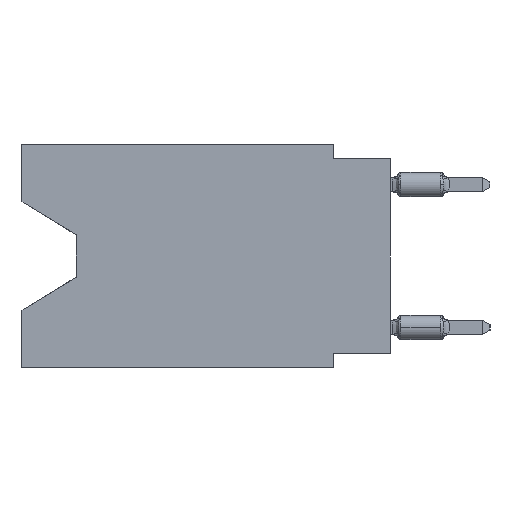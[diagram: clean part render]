
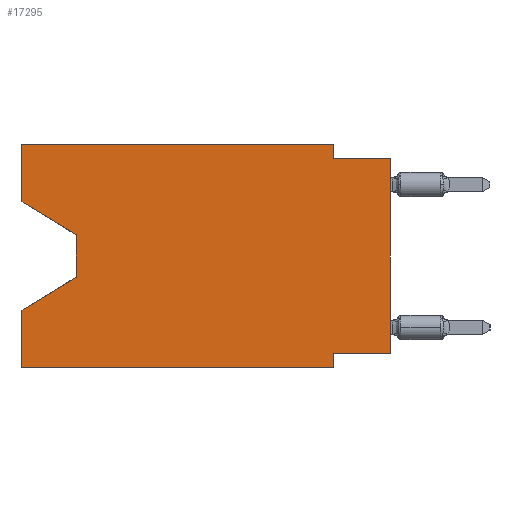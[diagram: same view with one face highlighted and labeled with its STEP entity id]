
A CAD part, left-side view. The second image highlights one B-rep face of the part: STEP entity #17295.
In plain terms, the highlighted planar face has unit normal (-1, 0, 0).
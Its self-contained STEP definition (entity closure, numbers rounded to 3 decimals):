
#108 = LINE ( 'NONE', #28120, #37864 ) ;
#518 = DIRECTION ( 'NONE',  ( 0., 0.855, -0.519 ) ) ;
#719 = DIRECTION ( 'NONE',  ( 1., 0., 0. ) ) ;
#915 = EDGE_CURVE ( 'NONE', #39426, #42097, #6991, .T. ) ;
#1503 = ORIENTED_EDGE ( 'NONE', *, *, #33979, .T. ) ;
#1703 = VECTOR ( 'NONE', #30741, 1000. ) ;
#4062 = ORIENTED_EDGE ( 'NONE', *, *, #31071, .F. ) ;
#4151 = VERTEX_POINT ( 'NONE', #44244 ) ;
#4306 = CARTESIAN_POINT ( 'NONE',  ( 0., 16.383, 0. ) ) ;
#4831 = CARTESIAN_POINT ( 'NONE',  ( 0., 16.383, 0. ) ) ;
#5642 = EDGE_CURVE ( 'NONE', #6560, #11931, #108, .T. ) ;
#6140 = LINE ( 'NONE', #20152, #36216 ) ;
#6560 = VERTEX_POINT ( 'NONE', #17883 ) ;
#6873 = ORIENTED_EDGE ( 'NONE', *, *, #22415, .T. ) ;
#6991 = LINE ( 'NONE', #17326, #15964 ) ;
#7248 = DIRECTION ( 'NONE',  ( 0., 0., 1. ) ) ;
#7378 = DIRECTION ( 'NONE',  ( 0., 0., -1. ) ) ;
#7526 = VECTOR ( 'NONE', #518, 1000. ) ;
#8379 = DIRECTION ( 'NONE',  ( 0., 0., 1. ) ) ;
#8474 = CARTESIAN_POINT ( 'NONE',  ( 0., 16.383, -9.906 ) ) ;
#8955 = DIRECTION ( 'NONE',  ( 0., -1., 0. ) ) ;
#9153 = ORIENTED_EDGE ( 'NONE', *, *, #14488, .F. ) ;
#10204 = CARTESIAN_POINT ( 'NONE',  ( 0., 2.54, -0.635 ) ) ;
#10482 = VECTOR ( 'NONE', #43753, 1000. ) ;
#10661 = VECTOR ( 'NONE', #20862, 1000. ) ;
#11818 = LINE ( 'NONE', #39403, #36347 ) ;
#11931 = VERTEX_POINT ( 'NONE', #4306 ) ;
#12626 = LINE ( 'NONE', #4831, #39075 ) ;
#13774 = ORIENTED_EDGE ( 'NONE', *, *, #33832, .F. ) ;
#13860 = EDGE_CURVE ( 'NONE', #42097, #24738, #31935, .T. ) ;
#14488 = EDGE_CURVE ( 'NONE', #4151, #15485, #6140, .T. ) ;
#15102 = CARTESIAN_POINT ( 'NONE',  ( 0., 2.54, -9.906 ) ) ;
#15473 = LINE ( 'NONE', #37067, #10482 ) ;
#15485 = VERTEX_POINT ( 'NONE', #10204 ) ;
#15964 = VECTOR ( 'NONE', #38912, 1000. ) ;
#16882 = AXIS2_PLACEMENT_3D ( 'NONE', #36060, #719, #7378 ) ;
#17088 = DIRECTION ( 'NONE',  ( 0., 0., -1. ) ) ;
#17162 = ORIENTED_EDGE ( 'NONE', *, *, #13860, .F. ) ;
#17295 = ADVANCED_FACE ( 'NONE', ( #29173 ), #39537, .F. ) ;
#17326 = CARTESIAN_POINT ( 'NONE',  ( 0., 0., -9.271 ) ) ;
#17883 = CARTESIAN_POINT ( 'NONE',  ( 0., 16.383, -2.546 ) ) ;
#17967 = CARTESIAN_POINT ( 'NONE',  ( 0., 13.97, -5.893 ) ) ;
#18507 = VERTEX_POINT ( 'NONE', #38573 ) ;
#19375 = VERTEX_POINT ( 'NONE', #31713 ) ;
#20152 = CARTESIAN_POINT ( 'NONE',  ( 0., 2.54, 0. ) ) ;
#20618 = CARTESIAN_POINT ( 'NONE',  ( 0., 0., -0.635 ) ) ;
#20635 = LINE ( 'NONE', #38099, #1703 ) ;
#20862 = DIRECTION ( 'NONE',  ( 0., -1., 0. ) ) ;
#21044 = LINE ( 'NONE', #38731, #32631 ) ;
#21822 = VERTEX_POINT ( 'NONE', #38479 ) ;
#22086 = EDGE_CURVE ( 'NONE', #18507, #37340, #15473, .T. ) ;
#22415 = EDGE_CURVE ( 'NONE', #37340, #19375, #24639, .T. ) ;
#22824 = ORIENTED_EDGE ( 'NONE', *, *, #5642, .F. ) ;
#22958 = ORIENTED_EDGE ( 'NONE', *, *, #32841, .F. ) ;
#23293 = CARTESIAN_POINT ( 'NONE',  ( 0., 13.97, -5.893 ) ) ;
#24530 = LINE ( 'NONE', #20618, #10661 ) ;
#24639 = LINE ( 'NONE', #17967, #7526 ) ;
#24738 = VERTEX_POINT ( 'NONE', #15102 ) ;
#24824 = CARTESIAN_POINT ( 'NONE',  ( 0., 2.54, -9.906 ) ) ;
#25557 = VECTOR ( 'NONE', #36490, 1000. ) ;
#25859 = ORIENTED_EDGE ( 'NONE', *, *, #32768, .T. ) ;
#27355 = CARTESIAN_POINT ( 'NONE',  ( 0., 2.54, -9.271 ) ) ;
#27859 = EDGE_LOOP ( 'NONE', ( #1503, #43008, #6873, #22958, #37829, #17162, #40151, #25859, #4062, #9153, #13774, #22824 ) ) ;
#28120 = CARTESIAN_POINT ( 'NONE',  ( 0., 16.383, 0. ) ) ;
#29173 = FACE_OUTER_BOUND ( 'NONE', #27859, .T. ) ;
#30741 = DIRECTION ( 'NONE',  ( 0., -0.855, -0.519 ) ) ;
#31071 = EDGE_CURVE ( 'NONE', #15485, #42994, #24530, .T. ) ;
#31713 = CARTESIAN_POINT ( 'NONE',  ( 0., 16.383, -7.36 ) ) ;
#31794 = VECTOR ( 'NONE', #17088, 1000. ) ;
#31935 = LINE ( 'NONE', #24824, #31794 ) ;
#32631 = VECTOR ( 'NONE', #7248, 1000. ) ;
#32768 = EDGE_CURVE ( 'NONE', #39426, #42994, #21044, .T. ) ;
#32841 = EDGE_CURVE ( 'NONE', #21822, #19375, #11818, .T. ) ;
#33832 = EDGE_CURVE ( 'NONE', #11931, #4151, #12626, .T. ) ;
#33918 = DIRECTION ( 'NONE',  ( 0., 0., -1. ) ) ;
#33979 = EDGE_CURVE ( 'NONE', #6560, #18507, #20635, .T. ) ;
#36060 = CARTESIAN_POINT ( 'NONE',  ( 0., 16.383, 0. ) ) ;
#36216 = VECTOR ( 'NONE', #33918, 1000. ) ;
#36347 = VECTOR ( 'NONE', #8379, 1000. ) ;
#36490 = DIRECTION ( 'NONE',  ( 0., -1., 0. ) ) ;
#37067 = CARTESIAN_POINT ( 'NONE',  ( 0., 13.97, -4.013 ) ) ;
#37340 = VERTEX_POINT ( 'NONE', #23293 ) ;
#37829 = ORIENTED_EDGE ( 'NONE', *, *, #42273, .T. ) ;
#37864 = VECTOR ( 'NONE', #42167, 1000. ) ;
#38099 = CARTESIAN_POINT ( 'NONE',  ( 0., 16.383, -2.546 ) ) ;
#38479 = CARTESIAN_POINT ( 'NONE',  ( 0., 16.383, -9.906 ) ) ;
#38573 = CARTESIAN_POINT ( 'NONE',  ( 0., 13.97, -4.013 ) ) ;
#38731 = CARTESIAN_POINT ( 'NONE',  ( 0., 0., 0. ) ) ;
#38912 = DIRECTION ( 'NONE',  ( 0., 1., 0. ) ) ;
#39075 = VECTOR ( 'NONE', #8955, 1000. ) ;
#39403 = CARTESIAN_POINT ( 'NONE',  ( 0., 16.383, 0. ) ) ;
#39426 = VERTEX_POINT ( 'NONE', #41667 ) ;
#39537 = PLANE ( 'NONE',  #16882 ) ;
#40151 = ORIENTED_EDGE ( 'NONE', *, *, #915, .F. ) ;
#40413 = LINE ( 'NONE', #8474, #25557 ) ;
#41667 = CARTESIAN_POINT ( 'NONE',  ( 0., 0., -9.271 ) ) ;
#42097 = VERTEX_POINT ( 'NONE', #27355 ) ;
#42167 = DIRECTION ( 'NONE',  ( 0., 0., 1. ) ) ;
#42273 = EDGE_CURVE ( 'NONE', #21822, #24738, #40413, .T. ) ;
#42994 = VERTEX_POINT ( 'NONE', #44332 ) ;
#43008 = ORIENTED_EDGE ( 'NONE', *, *, #22086, .T. ) ;
#43753 = DIRECTION ( 'NONE',  ( 0., 0., -1. ) ) ;
#44244 = CARTESIAN_POINT ( 'NONE',  ( 0., 2.54, 0. ) ) ;
#44332 = CARTESIAN_POINT ( 'NONE',  ( 0., 0., -0.635 ) ) ;
